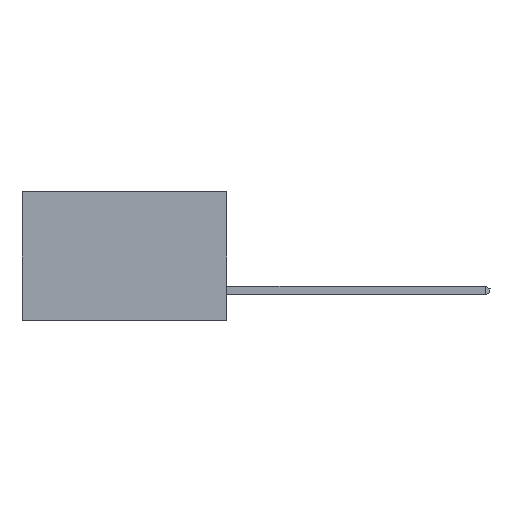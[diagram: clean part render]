
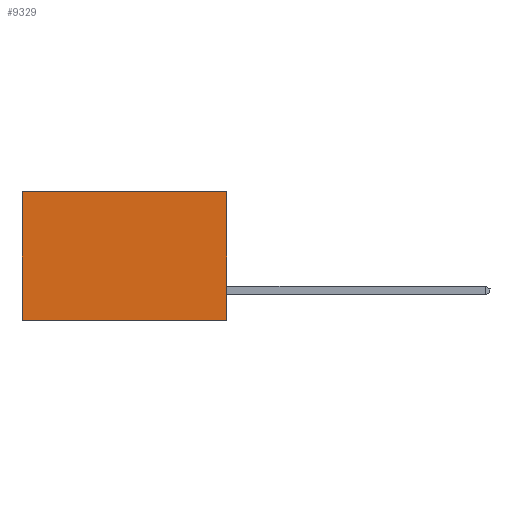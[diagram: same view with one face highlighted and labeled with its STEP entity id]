
A CAD part, left-side view. The second image highlights one B-rep face of the part: STEP entity #9329.
In plain terms, the highlighted planar face has unit normal (-1, 0, 0).
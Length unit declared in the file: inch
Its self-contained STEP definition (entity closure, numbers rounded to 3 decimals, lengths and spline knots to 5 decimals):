
#62 = VECTOR ( 'NONE', #10196, 39.37008 ) ;
#737 = VECTOR ( 'NONE', #8512, 39.37008 ) ;
#822 = CARTESIAN_POINT ( 'NONE',  ( 0.277, 0.59, -0.37 ) ) ;
#1181 = LINE ( 'NONE', #8638, #737 ) ;
#2283 = EDGE_CURVE ( 'NONE', #7154, #10670, #10739, .T. ) ;
#2389 = EDGE_CURVE ( 'NONE', #15844, #7154, #1181, .T. ) ;
#2733 = CARTESIAN_POINT ( 'NONE',  ( 0.277, 0.59, -0.37 ) ) ;
#3428 = ORIENTED_EDGE ( 'NONE', *, *, #2389, .F. ) ;
#3950 = AXIS2_PLACEMENT_3D ( 'NONE', #6246, #7477, #15586 ) ;
#4049 = ORIENTED_EDGE ( 'NONE', *, *, #14453, .T. ) ;
#5157 = ORIENTED_EDGE ( 'NONE', *, *, #2283, .F. ) ;
#5560 = LINE ( 'NONE', #822, #11598 ) ;
#5883 = CARTESIAN_POINT ( 'NONE',  ( 0.277, 0., 0. ) ) ;
#6246 = CARTESIAN_POINT ( 'NONE',  ( 0.277, 0., -0.37 ) ) ;
#6625 = ORIENTED_EDGE ( 'NONE', *, *, #8518, .T. ) ;
#7154 = VERTEX_POINT ( 'NONE', #11359 ) ;
#7435 = PLANE ( 'NONE',  #3950 ) ;
#7477 = DIRECTION ( 'NONE',  ( 1., 0., 0. ) ) ;
#7841 = FACE_OUTER_BOUND ( 'NONE', #7916, .T. ) ;
#7862 = VECTOR ( 'NONE', #13042, 39.37008 ) ;
#7916 = EDGE_LOOP ( 'NONE', ( #6625, #5157, #3428, #4049 ) ) ;
#8512 = DIRECTION ( 'NONE',  ( 0., 0., -1. ) ) ;
#8518 = EDGE_CURVE ( 'NONE', #14406, #10670, #5560, .T. ) ;
#8638 = CARTESIAN_POINT ( 'NONE',  ( 0.277, 0., -0.37 ) ) ;
#9329 = ADVANCED_FACE ( 'NONE', ( #7841 ), #7435, .F. ) ;
#9820 = DIRECTION ( 'NONE',  ( 0., 0., -1. ) ) ;
#10196 = DIRECTION ( 'NONE',  ( 0., 1., 0. ) ) ;
#10352 = CARTESIAN_POINT ( 'NONE',  ( 0.277, 0., -0.37 ) ) ;
#10670 = VERTEX_POINT ( 'NONE', #2733 ) ;
#10739 = LINE ( 'NONE', #10352, #62 ) ;
#11359 = CARTESIAN_POINT ( 'NONE',  ( 0.277, 0., -0.37 ) ) ;
#11598 = VECTOR ( 'NONE', #9820, 39.37008 ) ;
#11828 = CARTESIAN_POINT ( 'NONE',  ( 0.277, 0.59, 0. ) ) ;
#12860 = CARTESIAN_POINT ( 'NONE',  ( 0.277, 0., 0. ) ) ;
#13042 = DIRECTION ( 'NONE',  ( 0., 1., 0. ) ) ;
#14095 = LINE ( 'NONE', #5883, #7862 ) ;
#14406 = VERTEX_POINT ( 'NONE', #11828 ) ;
#14453 = EDGE_CURVE ( 'NONE', #15844, #14406, #14095, .T. ) ;
#15586 = DIRECTION ( 'NONE',  ( 0., 0., -1. ) ) ;
#15844 = VERTEX_POINT ( 'NONE', #12860 ) ;
